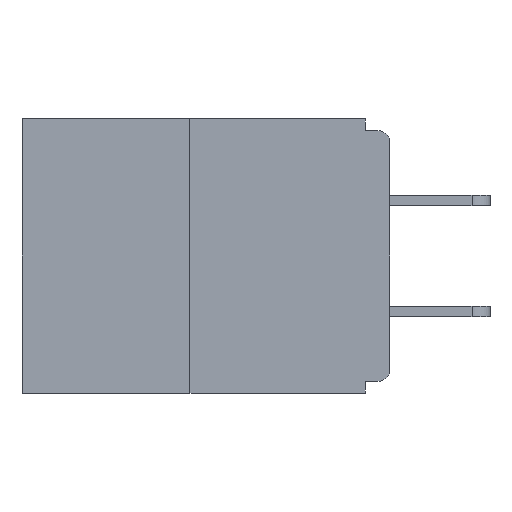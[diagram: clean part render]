
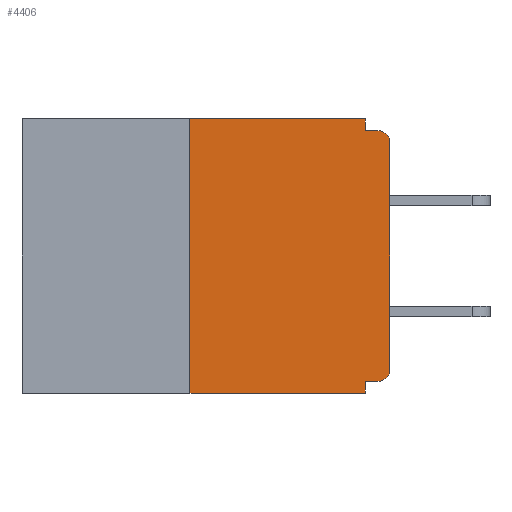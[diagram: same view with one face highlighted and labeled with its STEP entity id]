
A CAD part, left-side view. The second image highlights one B-rep face of the part: STEP entity #4406.
In plain terms, the highlighted planar face has unit normal (-1, 0, 0).
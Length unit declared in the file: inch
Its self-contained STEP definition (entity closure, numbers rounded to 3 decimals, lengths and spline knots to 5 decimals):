
#778 = AXIS2_PLACEMENT_3D ( 'NONE', #9602, #6157, #5990 ) ;
#832 = ORIENTED_EDGE ( 'NONE', *, *, #6138, .T. ) ;
#1016 = EDGE_CURVE ( 'NONE', #8292, #10108, #14292, .T. ) ;
#1449 = ORIENTED_EDGE ( 'NONE', *, *, #15851, .F. ) ;
#1502 = CARTESIAN_POINT ( 'NONE',  ( 0., 0.031, -0.343 ) ) ;
#1536 = VERTEX_POINT ( 'NONE', #6079 ) ;
#1647 = LINE ( 'NONE', #1502, #14032 ) ;
#1892 = VECTOR ( 'NONE', #3801, 39.37008 ) ;
#2007 = ORIENTED_EDGE ( 'NONE', *, *, #8885, .T. ) ;
#2053 = VECTOR ( 'NONE', #15141, 39.37008 ) ;
#2075 = EDGE_CURVE ( 'NONE', #8010, #10909, #14057, .T. ) ;
#2528 = CARTESIAN_POINT ( 'NONE',  ( 0., 0.46, 0. ) ) ;
#2665 = CARTESIAN_POINT ( 'NONE',  ( 0., 0.031, -0.328 ) ) ;
#3143 = EDGE_CURVE ( 'NONE', #11115, #1536, #14638, .T. ) ;
#3297 = ORIENTED_EDGE ( 'NONE', *, *, #13360, .T. ) ;
#3697 = CARTESIAN_POINT ( 'NONE',  ( 0., 0.25, 0. ) ) ;
#3764 = VECTOR ( 'NONE', #16329, 39.37008 ) ;
#3801 = DIRECTION ( 'NONE',  ( 0., 0., 1. ) ) ;
#3803 = DIRECTION ( 'NONE',  ( 0., 0., -1. ) ) ;
#3866 = ORIENTED_EDGE ( 'NONE', *, *, #8312, .F. ) ;
#4237 = DIRECTION ( 'NONE',  ( 0., 0., -1. ) ) ;
#4406 = ADVANCED_FACE ( 'NONE', ( #15772 ), #8422, .F. ) ;
#4730 = ORIENTED_EDGE ( 'NONE', *, *, #7803, .F. ) ;
#4828 = VECTOR ( 'NONE', #3803, 39.37008 ) ;
#4890 = LINE ( 'NONE', #11460, #1892 ) ;
#5318 = CIRCLE ( 'NONE', #778, 0.015 ) ;
#5415 = DIRECTION ( 'NONE',  ( 0., -1., 0. ) ) ;
#5426 = VERTEX_POINT ( 'NONE', #14582 ) ;
#5437 = CARTESIAN_POINT ( 'NONE',  ( 0., 0.25, -0.343 ) ) ;
#5678 = VECTOR ( 'NONE', #12629, 39.37008 ) ;
#5732 = CARTESIAN_POINT ( 'NONE',  ( 0., 0.46, 0. ) ) ;
#5990 = DIRECTION ( 'NONE',  ( 0., 0., -1. ) ) ;
#6079 = CARTESIAN_POINT ( 'NONE',  ( 0., 0.25, 0. ) ) ;
#6138 = EDGE_CURVE ( 'NONE', #11115, #8392, #16120, .T. ) ;
#6157 = DIRECTION ( 'NONE',  ( -1., 0., 0. ) ) ;
#7274 = VERTEX_POINT ( 'NONE', #16028 ) ;
#7445 = CARTESIAN_POINT ( 'NONE',  ( 0., 0.015, -0.015 ) ) ;
#7484 = CARTESIAN_POINT ( 'NONE',  ( 0., 0.015, -0.328 ) ) ;
#7613 = ORIENTED_EDGE ( 'NONE', *, *, #10020, .T. ) ;
#7743 = ORIENTED_EDGE ( 'NONE', *, *, #1016, .F. ) ;
#7803 = EDGE_CURVE ( 'NONE', #10108, #8392, #1647, .T. ) ;
#8010 = VERTEX_POINT ( 'NONE', #10722 ) ;
#8292 = VERTEX_POINT ( 'NONE', #7484 ) ;
#8312 = EDGE_CURVE ( 'NONE', #1536, #7274, #9271, .T. ) ;
#8392 = VERTEX_POINT ( 'NONE', #12872 ) ;
#8422 = PLANE ( 'NONE',  #10879 ) ;
#8885 = EDGE_CURVE ( 'NONE', #8292, #13808, #14405, .T. ) ;
#9271 = LINE ( 'NONE', #2528, #2053 ) ;
#9602 = CARTESIAN_POINT ( 'NONE',  ( 0., 0.015, -0.03 ) ) ;
#9897 = DIRECTION ( 'NONE',  ( -1., 0., 0. ) ) ;
#10020 = EDGE_CURVE ( 'NONE', #5426, #10909, #5318, .T. ) ;
#10108 = VERTEX_POINT ( 'NONE', #2665 ) ;
#10722 = CARTESIAN_POINT ( 'NONE',  ( 0., 0.031, -0.015 ) ) ;
#10744 = VECTOR ( 'NONE', #12107, 39.37008 ) ;
#10879 = AXIS2_PLACEMENT_3D ( 'NONE', #5732, #15876, #14630 ) ;
#10909 = VERTEX_POINT ( 'NONE', #7445 ) ;
#11115 = VERTEX_POINT ( 'NONE', #5437 ) ;
#11134 = CARTESIAN_POINT ( 'NONE',  ( 0., 0.015, -0.313 ) ) ;
#11460 = CARTESIAN_POINT ( 'NONE',  ( 0., 0., 0. ) ) ;
#12028 = ORIENTED_EDGE ( 'NONE', *, *, #2075, .F. ) ;
#12103 = CARTESIAN_POINT ( 'NONE',  ( 0., 0., -0.313 ) ) ;
#12107 = DIRECTION ( 'NONE',  ( 0., -1., 0. ) ) ;
#12167 = VECTOR ( 'NONE', #5415, 39.37008 ) ;
#12564 = DIRECTION ( 'NONE',  ( 0., 0., -1. ) ) ;
#12629 = DIRECTION ( 'NONE',  ( 0., 0., 1. ) ) ;
#12726 = CARTESIAN_POINT ( 'NONE',  ( 0., 0.031, 0. ) ) ;
#12872 = CARTESIAN_POINT ( 'NONE',  ( 0., 0.031, -0.343 ) ) ;
#13360 = EDGE_CURVE ( 'NONE', #13808, #5426, #4890, .T. ) ;
#13437 = AXIS2_PLACEMENT_3D ( 'NONE', #11134, #9897, #12564 ) ;
#13442 = CARTESIAN_POINT ( 'NONE',  ( 0., 0., -0.015 ) ) ;
#13476 = ORIENTED_EDGE ( 'NONE', *, *, #3143, .F. ) ;
#13516 = EDGE_LOOP ( 'NONE', ( #3866, #13476, #832, #4730, #7743, #2007, #3297, #7613, #12028, #1449 ) ) ;
#13740 = CARTESIAN_POINT ( 'NONE',  ( 0., 0., -0.328 ) ) ;
#13808 = VERTEX_POINT ( 'NONE', #12103 ) ;
#14032 = VECTOR ( 'NONE', #4237, 39.37008 ) ;
#14057 = LINE ( 'NONE', #13442, #10744 ) ;
#14202 = CARTESIAN_POINT ( 'NONE',  ( 0., 0.46, -0.343 ) ) ;
#14292 = LINE ( 'NONE', #13740, #3764 ) ;
#14405 = CIRCLE ( 'NONE', #13437, 0.015 ) ;
#14582 = CARTESIAN_POINT ( 'NONE',  ( 0., 0., -0.03 ) ) ;
#14630 = DIRECTION ( 'NONE',  ( 0., 0., -1. ) ) ;
#14638 = LINE ( 'NONE', #3697, #5678 ) ;
#14978 = LINE ( 'NONE', #12726, #4828 ) ;
#15141 = DIRECTION ( 'NONE',  ( 0., -1., 0. ) ) ;
#15772 = FACE_OUTER_BOUND ( 'NONE', #13516, .T. ) ;
#15851 = EDGE_CURVE ( 'NONE', #7274, #8010, #14978, .T. ) ;
#15876 = DIRECTION ( 'NONE',  ( 1., 0., 0. ) ) ;
#16028 = CARTESIAN_POINT ( 'NONE',  ( 0., 0.031, 0. ) ) ;
#16120 = LINE ( 'NONE', #14202, #12167 ) ;
#16329 = DIRECTION ( 'NONE',  ( 0., 1., 0. ) ) ;
